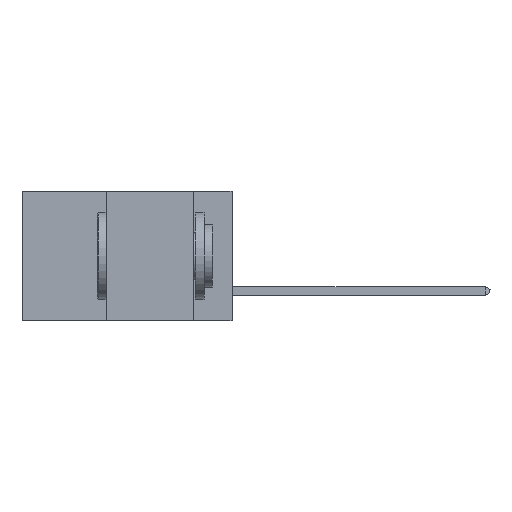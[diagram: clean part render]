
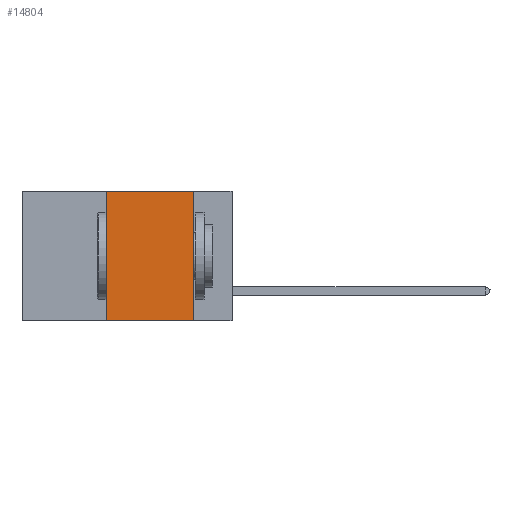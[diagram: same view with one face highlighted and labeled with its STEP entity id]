
A CAD part, left-side view. The second image highlights one B-rep face of the part: STEP entity #14804.
In plain terms, the highlighted planar face has unit normal (-1, 0, 0).
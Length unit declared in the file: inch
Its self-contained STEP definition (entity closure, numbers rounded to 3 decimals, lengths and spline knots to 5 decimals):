
#220 = FACE_OUTER_BOUND ( 'NONE', #3300, .T. ) ;
#359 = LINE ( 'NONE', #3450, #14412 ) ;
#824 = VERTEX_POINT ( 'NONE', #21747 ) ;
#1445 = EDGE_CURVE ( 'NONE', #3103, #10145, #9941, .T. ) ;
#2029 = CARTESIAN_POINT ( 'NONE',  ( 0., 0.6, 0. ) ) ;
#2308 = ORIENTED_EDGE ( 'NONE', *, *, #1445, .F. ) ;
#3103 = VERTEX_POINT ( 'NONE', #5681 ) ;
#3300 = EDGE_LOOP ( 'NONE', ( #2308, #15622, #9402, #11041 ) ) ;
#3450 = CARTESIAN_POINT ( 'NONE',  ( 0., 0.6, 0. ) ) ;
#4034 = DIRECTION ( 'NONE',  ( 1., 0., 0. ) ) ;
#4428 = LINE ( 'NONE', #22518, #13083 ) ;
#5681 = CARTESIAN_POINT ( 'NONE',  ( 0., 0.11, 0. ) ) ;
#5778 = CARTESIAN_POINT ( 'NONE',  ( 0., 0.11, -0.37 ) ) ;
#5850 = DIRECTION ( 'NONE',  ( 0., 0., -1. ) ) ;
#7336 = CARTESIAN_POINT ( 'NONE',  ( 0., 0.36, -0.37 ) ) ;
#8179 = CARTESIAN_POINT ( 'NONE',  ( 0., 0.6, -0.37 ) ) ;
#8354 = EDGE_CURVE ( 'NONE', #16270, #824, #4428, .T. ) ;
#8797 = CARTESIAN_POINT ( 'NONE',  ( 0., 0.11, 0. ) ) ;
#9003 = DIRECTION ( 'NONE',  ( 0., -1., 0. ) ) ;
#9402 = ORIENTED_EDGE ( 'NONE', *, *, #8354, .F. ) ;
#9941 = LINE ( 'NONE', #8797, #12028 ) ;
#10145 = VERTEX_POINT ( 'NONE', #5778 ) ;
#10865 = DIRECTION ( 'NONE',  ( 0., 0., -1. ) ) ;
#11041 = ORIENTED_EDGE ( 'NONE', *, *, #14830, .T. ) ;
#12028 = VECTOR ( 'NONE', #10865, 39.37008 ) ;
#12369 = EDGE_CURVE ( 'NONE', #824, #3103, #359, .T. ) ;
#13083 = VECTOR ( 'NONE', #24699, 39.37008 ) ;
#14412 = VECTOR ( 'NONE', #9003, 39.37008 ) ;
#14804 = ADVANCED_FACE ( 'NONE', ( #220 ), #23151, .F. ) ;
#14830 = EDGE_CURVE ( 'NONE', #16270, #10145, #23586, .T. ) ;
#15622 = ORIENTED_EDGE ( 'NONE', *, *, #12369, .F. ) ;
#16270 = VERTEX_POINT ( 'NONE', #7336 ) ;
#19998 = VECTOR ( 'NONE', #21728, 39.37008 ) ;
#20201 = AXIS2_PLACEMENT_3D ( 'NONE', #2029, #4034, #5850 ) ;
#21728 = DIRECTION ( 'NONE',  ( 0., -1., 0. ) ) ;
#21747 = CARTESIAN_POINT ( 'NONE',  ( 0., 0.36, 0. ) ) ;
#22518 = CARTESIAN_POINT ( 'NONE',  ( 0., 0.36, 0. ) ) ;
#23151 = PLANE ( 'NONE',  #20201 ) ;
#23586 = LINE ( 'NONE', #8179, #19998 ) ;
#24699 = DIRECTION ( 'NONE',  ( 0., 0., 1. ) ) ;
